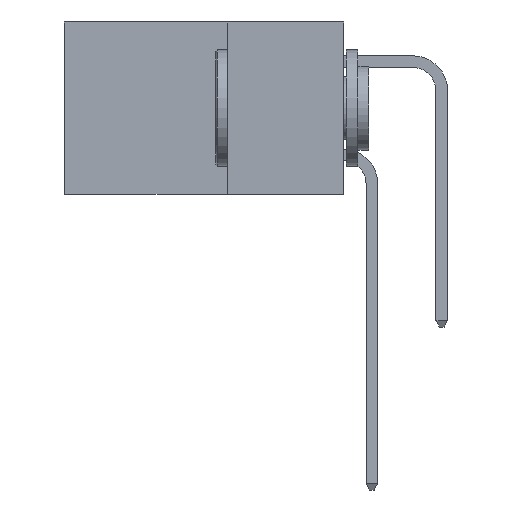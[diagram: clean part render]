
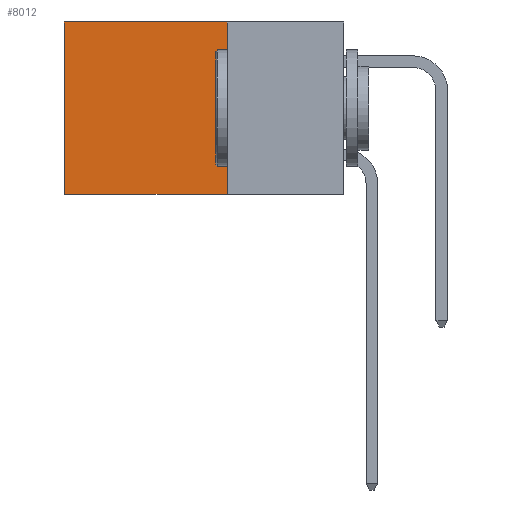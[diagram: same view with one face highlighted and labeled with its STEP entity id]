
A CAD part, left-side view. The second image highlights one B-rep face of the part: STEP entity #8012.
In plain terms, the highlighted planar face has unit normal (-1, 0, 0).
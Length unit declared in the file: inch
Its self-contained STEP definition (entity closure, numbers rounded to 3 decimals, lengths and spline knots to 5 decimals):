
#821 = EDGE_LOOP ( 'NONE', ( #7631, #22713, #15583, #11478 ) ) ;
#1774 = PLANE ( 'NONE',  #24215 ) ;
#3004 = EDGE_CURVE ( 'NONE', #15176, #13196, #17080, .T. ) ;
#3125 = LINE ( 'NONE', #4164, #25255 ) ;
#3471 = LINE ( 'NONE', #5079, #13496 ) ;
#3931 = DIRECTION ( 'NONE',  ( 0., 0., -1. ) ) ;
#4164 = CARTESIAN_POINT ( 'NONE',  ( 0.2615, 0.6, -0.37 ) ) ;
#5079 = CARTESIAN_POINT ( 'NONE',  ( 0.2615, 0.25, 0. ) ) ;
#7631 = ORIENTED_EDGE ( 'NONE', *, *, #17911, .T. ) ;
#8012 = ADVANCED_FACE ( 'NONE', ( #24298 ), #1774, .F. ) ;
#8442 = DIRECTION ( 'NONE',  ( 0., 0., -1. ) ) ;
#11478 = ORIENTED_EDGE ( 'NONE', *, *, #13769, .T. ) ;
#11671 = CARTESIAN_POINT ( 'NONE',  ( 0.2615, 0.6, -0.37 ) ) ;
#12214 = VERTEX_POINT ( 'NONE', #19240 ) ;
#13196 = VERTEX_POINT ( 'NONE', #11671 ) ;
#13496 = VECTOR ( 'NONE', #24372, 39.37008 ) ;
#13769 = EDGE_CURVE ( 'NONE', #12214, #14800, #3471, .T. ) ;
#14800 = VERTEX_POINT ( 'NONE', #26226 ) ;
#15176 = VERTEX_POINT ( 'NONE', #20311 ) ;
#15244 = CARTESIAN_POINT ( 'NONE',  ( 0.2615, 0.25, -0.37 ) ) ;
#15509 = DIRECTION ( 'NONE',  ( 0., 1., 0. ) ) ;
#15583 = ORIENTED_EDGE ( 'NONE', *, *, #20357, .F. ) ;
#16727 = DIRECTION ( 'NONE',  ( 1., 0., 0. ) ) ;
#16849 = CARTESIAN_POINT ( 'NONE',  ( 0.2615, 0.25, -0.37 ) ) ;
#17080 = LINE ( 'NONE', #15244, #22823 ) ;
#17911 = EDGE_CURVE ( 'NONE', #14800, #13196, #3125, .T. ) ;
#19240 = CARTESIAN_POINT ( 'NONE',  ( 0.2615, 0.25, 0. ) ) ;
#20311 = CARTESIAN_POINT ( 'NONE',  ( 0.2615, 0.25, -0.37 ) ) ;
#20357 = EDGE_CURVE ( 'NONE', #12214, #15176, #27102, .T. ) ;
#21422 = VECTOR ( 'NONE', #8442, 39.37008 ) ;
#22713 = ORIENTED_EDGE ( 'NONE', *, *, #3004, .F. ) ;
#22823 = VECTOR ( 'NONE', #15509, 39.37008 ) ;
#23127 = CARTESIAN_POINT ( 'NONE',  ( 0.2615, 0.25, -0.37 ) ) ;
#23445 = DIRECTION ( 'NONE',  ( 0., 0., -1. ) ) ;
#24215 = AXIS2_PLACEMENT_3D ( 'NONE', #23127, #16727, #3931 ) ;
#24298 = FACE_OUTER_BOUND ( 'NONE', #821, .T. ) ;
#24372 = DIRECTION ( 'NONE',  ( 0., 1., 0. ) ) ;
#25255 = VECTOR ( 'NONE', #23445, 39.37008 ) ;
#26226 = CARTESIAN_POINT ( 'NONE',  ( 0.2615, 0.6, 0. ) ) ;
#27102 = LINE ( 'NONE', #16849, #21422 ) ;
